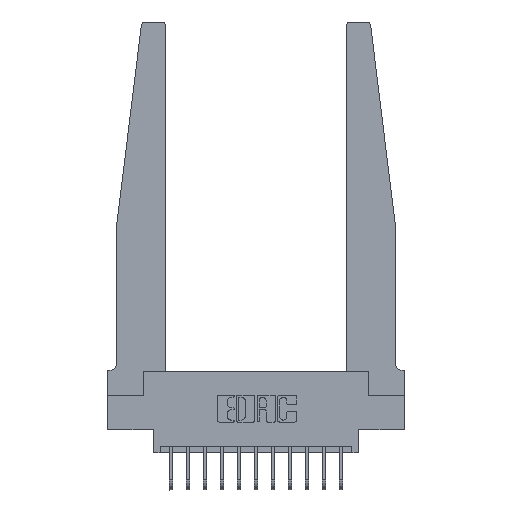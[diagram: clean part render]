
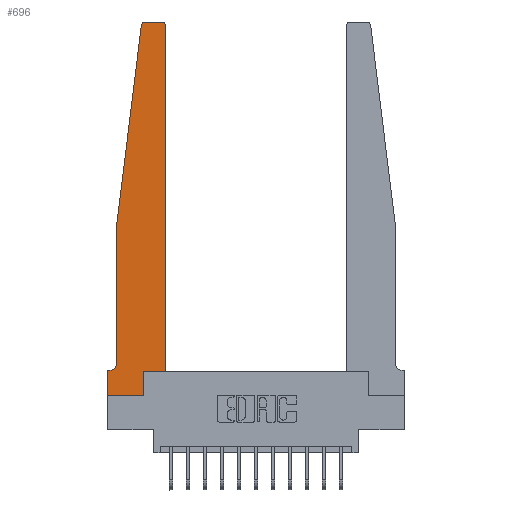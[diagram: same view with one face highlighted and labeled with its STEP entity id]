
A CAD part, top view. The second image highlights one B-rep face of the part: STEP entity #696.
In plain terms, the highlighted planar face has unit normal (0, 0, 1).
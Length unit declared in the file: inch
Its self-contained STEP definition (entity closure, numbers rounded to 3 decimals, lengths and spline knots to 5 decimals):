
#27 = VECTOR ( 'NONE', #1550, 39.37008 ) ;
#116 = ORIENTED_EDGE ( 'NONE', *, *, #11324, .T. ) ;
#257 = VECTOR ( 'NONE', #17905, 39.37008 ) ;
#336 = CARTESIAN_POINT ( 'NONE',  ( 0.065, 1.25, 0.37 ) ) ;
#508 = DIRECTION ( 'NONE',  ( -0.122, -0.992, 0. ) ) ;
#696 = ADVANCED_FACE ( 'NONE', ( #6812 ), #15043, .T. ) ;
#809 = CARTESIAN_POINT ( 'NONE',  ( 0.24675, 2.72367, 0.37 ) ) ;
#1208 = CIRCLE ( 'NONE', #11528, 0.03 ) ;
#1500 = DIRECTION ( 'NONE',  ( 1., 0., 0. ) ) ;
#1550 = DIRECTION ( 'NONE',  ( -1., 0., 0. ) ) ;
#1626 = CARTESIAN_POINT ( 'NONE',  ( 0.27653, 2.72, 0.37 ) ) ;
#1667 = VERTEX_POINT ( 'NONE', #13043 ) ;
#1906 = VERTEX_POINT ( 'NONE', #16043 ) ;
#1998 = EDGE_CURVE ( 'NONE', #11814, #14469, #10760, .T. ) ;
#2336 = CARTESIAN_POINT ( 'NONE',  ( 0.015, 0.2375, 0.37 ) ) ;
#2384 = LINE ( 'NONE', #6927, #16761 ) ;
#2470 = VERTEX_POINT ( 'NONE', #3692 ) ;
#2518 = DIRECTION ( 'NONE',  ( 0., 0., -1. ) ) ;
#2629 = EDGE_CURVE ( 'NONE', #8999, #10362, #16156, .T. ) ;
#3202 = EDGE_CURVE ( 'NONE', #1667, #8999, #14623, .T. ) ;
#3206 = AXIS2_PLACEMENT_3D ( 'NONE', #10941, #16475, #12230 ) ;
#3359 = DIRECTION ( 'NONE',  ( 1., 0., 0. ) ) ;
#3640 = EDGE_CURVE ( 'NONE', #2470, #1906, #8495, .T. ) ;
#3676 = LINE ( 'NONE', #10224, #6051 ) ;
#3692 = CARTESIAN_POINT ( 'NONE',  ( 0.2605, 0.18, 0.37 ) ) ;
#3716 = CARTESIAN_POINT ( 'NONE',  ( 0.015, 0.1875, 0.37 ) ) ;
#4096 = DIRECTION ( 'NONE',  ( 0., 1., 0. ) ) ;
#4515 = AXIS2_PLACEMENT_3D ( 'NONE', #2336, #2518, #5068 ) ;
#4599 = AXIS2_PLACEMENT_3D ( 'NONE', #6664, #12318, #5326 ) ;
#5025 = VECTOR ( 'NONE', #4096, 39.37008 ) ;
#5068 = DIRECTION ( 'NONE',  ( -1., 0., 0. ) ) ;
#5326 = DIRECTION ( 'NONE',  ( 1., 0., 0. ) ) ;
#5349 = ORIENTED_EDGE ( 'NONE', *, *, #11413, .T. ) ;
#5404 = VERTEX_POINT ( 'NONE', #9965 ) ;
#5772 = CARTESIAN_POINT ( 'NONE',  ( 0.425, 0.18, 0.37 ) ) ;
#6051 = VECTOR ( 'NONE', #3359, 39.37008 ) ;
#6419 = ORIENTED_EDGE ( 'NONE', *, *, #3640, .T. ) ;
#6664 = CARTESIAN_POINT ( 'NONE',  ( 0., 0.1875, 0.37 ) ) ;
#6764 = VECTOR ( 'NONE', #13585, 39.37008 ) ;
#6794 = CARTESIAN_POINT ( 'NONE',  ( 0.25, 2.75, 0.37 ) ) ;
#6812 = FACE_OUTER_BOUND ( 'NONE', #16640, .T. ) ;
#6824 = CARTESIAN_POINT ( 'NONE',  ( 0.27653, 2.75, 0.37 ) ) ;
#6927 = CARTESIAN_POINT ( 'NONE',  ( 0.065, 1.25, 0.37 ) ) ;
#6996 = LINE ( 'NONE', #336, #9442 ) ;
#7140 = VERTEX_POINT ( 'NONE', #11664 ) ;
#8006 = CARTESIAN_POINT ( 'NONE',  ( 0., 0.1875, 0.37 ) ) ;
#8040 = DIRECTION ( 'NONE',  ( 1., 0., 0. ) ) ;
#8068 = CARTESIAN_POINT ( 'NONE',  ( 0., 0., 0.37 ) ) ;
#8399 = ORIENTED_EDGE ( 'NONE', *, *, #14249, .T. ) ;
#8495 = LINE ( 'NONE', #17642, #11314 ) ;
#8518 = EDGE_CURVE ( 'NONE', #1906, #7140, #9043, .T. ) ;
#8753 = LINE ( 'NONE', #16630, #5025 ) ;
#8999 = VERTEX_POINT ( 'NONE', #3716 ) ;
#9043 = LINE ( 'NONE', #5772, #17986 ) ;
#9137 = CIRCLE ( 'NONE', #3206, 0.03 ) ;
#9156 = CARTESIAN_POINT ( 'NONE',  ( 0.2605, 0., 0.37 ) ) ;
#9442 = VECTOR ( 'NONE', #15813, 39.37008 ) ;
#9490 = EDGE_CURVE ( 'NONE', #5404, #1667, #6996, .T. ) ;
#9965 = CARTESIAN_POINT ( 'NONE',  ( 0.065, 1.25, 0.37 ) ) ;
#10224 = CARTESIAN_POINT ( 'NONE',  ( 0., 0., 0.37 ) ) ;
#10304 = ORIENTED_EDGE ( 'NONE', *, *, #9490, .T. ) ;
#10308 = ORIENTED_EDGE ( 'NONE', *, *, #16841, .T. ) ;
#10362 = VERTEX_POINT ( 'NONE', #8006 ) ;
#10526 = CARTESIAN_POINT ( 'NONE',  ( 0., 0., 0.37 ) ) ;
#10760 = LINE ( 'NONE', #6794, #6764 ) ;
#10941 = CARTESIAN_POINT ( 'NONE',  ( 0.395, 2.72, 0.37 ) ) ;
#11314 = VECTOR ( 'NONE', #8040, 39.37008 ) ;
#11324 = EDGE_CURVE ( 'NONE', #17803, #16593, #3676, .T. ) ;
#11391 = ORIENTED_EDGE ( 'NONE', *, *, #13028, .T. ) ;
#11413 = EDGE_CURVE ( 'NONE', #12718, #5404, #2384, .T. ) ;
#11528 = AXIS2_PLACEMENT_3D ( 'NONE', #1626, #12554, #1500 ) ;
#11664 = CARTESIAN_POINT ( 'NONE',  ( 0.425, 2.72, 0.37 ) ) ;
#11814 = VERTEX_POINT ( 'NONE', #14562 ) ;
#12230 = DIRECTION ( 'NONE',  ( 1., 0., 0. ) ) ;
#12318 = DIRECTION ( 'NONE',  ( 0., 0., 1. ) ) ;
#12554 = DIRECTION ( 'NONE',  ( 0., 0., 1. ) ) ;
#12718 = VERTEX_POINT ( 'NONE', #809 ) ;
#13028 = EDGE_CURVE ( 'NONE', #7140, #11814, #9137, .T. ) ;
#13043 = CARTESIAN_POINT ( 'NONE',  ( 0.065, 0.2375, 0.37 ) ) ;
#13585 = DIRECTION ( 'NONE',  ( -1., 0., 0. ) ) ;
#13670 = ORIENTED_EDGE ( 'NONE', *, *, #3202, .T. ) ;
#13674 = CARTESIAN_POINT ( 'NONE',  ( 0.065, 0.1875, 0.37 ) ) ;
#13825 = EDGE_CURVE ( 'NONE', #14469, #12718, #1208, .T. ) ;
#14249 = EDGE_CURVE ( 'NONE', #10362, #17803, #16851, .T. ) ;
#14400 = ORIENTED_EDGE ( 'NONE', *, *, #8518, .T. ) ;
#14469 = VERTEX_POINT ( 'NONE', #6824 ) ;
#14562 = CARTESIAN_POINT ( 'NONE',  ( 0.395, 2.75, 0.37 ) ) ;
#14623 = CIRCLE ( 'NONE', #4515, 0.05 ) ;
#14634 = ORIENTED_EDGE ( 'NONE', *, *, #13825, .T. ) ;
#15043 = PLANE ( 'NONE',  #4599 ) ;
#15544 = DIRECTION ( 'NONE',  ( 0., 1., 0. ) ) ;
#15813 = DIRECTION ( 'NONE',  ( 0., -1., 0. ) ) ;
#15994 = ORIENTED_EDGE ( 'NONE', *, *, #2629, .T. ) ;
#16043 = CARTESIAN_POINT ( 'NONE',  ( 0.425, 0.18, 0.37 ) ) ;
#16156 = LINE ( 'NONE', #13674, #27 ) ;
#16449 = ORIENTED_EDGE ( 'NONE', *, *, #1998, .T. ) ;
#16475 = DIRECTION ( 'NONE',  ( 0., 0., 1. ) ) ;
#16593 = VERTEX_POINT ( 'NONE', #9156 ) ;
#16630 = CARTESIAN_POINT ( 'NONE',  ( 0.2605, 0.18, 0.37 ) ) ;
#16640 = EDGE_LOOP ( 'NONE', ( #16449, #14634, #5349, #10304, #13670, #15994, #8399, #116, #10308, #6419, #14400, #11391 ) ) ;
#16761 = VECTOR ( 'NONE', #508, 39.37008 ) ;
#16841 = EDGE_CURVE ( 'NONE', #16593, #2470, #8753, .T. ) ;
#16851 = LINE ( 'NONE', #8068, #257 ) ;
#17642 = CARTESIAN_POINT ( 'NONE',  ( 0.425, 0.18, 0.37 ) ) ;
#17803 = VERTEX_POINT ( 'NONE', #10526 ) ;
#17905 = DIRECTION ( 'NONE',  ( 0., -1., 0. ) ) ;
#17986 = VECTOR ( 'NONE', #15544, 39.37008 ) ;
